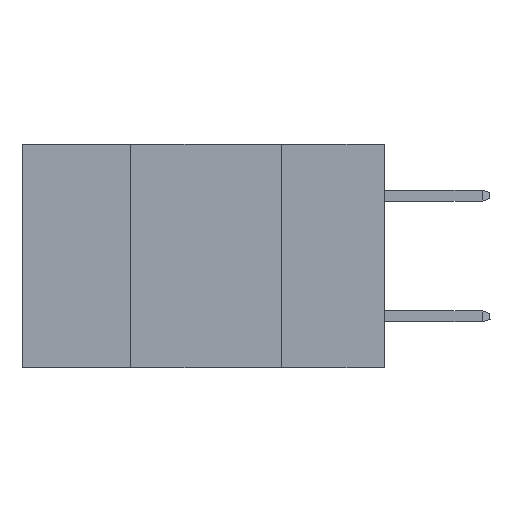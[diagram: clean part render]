
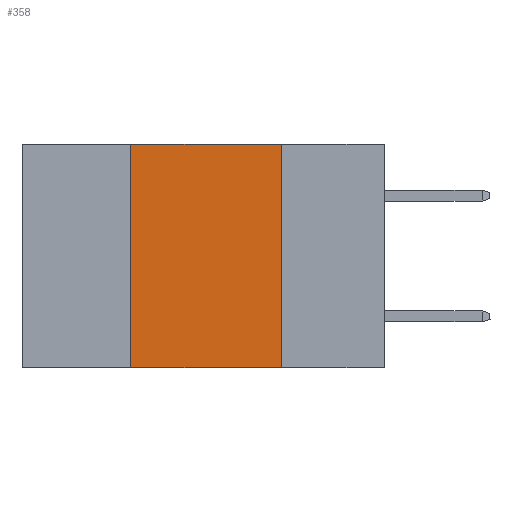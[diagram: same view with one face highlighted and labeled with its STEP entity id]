
A CAD part, left-side view. The second image highlights one B-rep face of the part: STEP entity #358.
In plain terms, the highlighted planar face has unit normal (-1, 0, 0).
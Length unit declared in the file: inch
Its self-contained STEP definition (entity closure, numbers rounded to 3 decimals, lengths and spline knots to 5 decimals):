
#71 = DIRECTION ( 'NONE',  ( 0., 0., -1. ) ) ;
#165 = CARTESIAN_POINT ( 'NONE',  ( 0., 0.42, -0.37 ) ) ;
#358 = ADVANCED_FACE ( 'NONE', ( #16092 ), #9782, .F. ) ;
#879 = VERTEX_POINT ( 'NONE', #4631 ) ;
#892 = DIRECTION ( 'NONE',  ( 0., -1., 0. ) ) ;
#1487 = CARTESIAN_POINT ( 'NONE',  ( 0., 0.17, -0.37 ) ) ;
#1535 = EDGE_CURVE ( 'NONE', #8017, #879, #15517, .T. ) ;
#1613 = DIRECTION ( 'NONE',  ( 0., 0., -1. ) ) ;
#1694 = AXIS2_PLACEMENT_3D ( 'NONE', #3619, #3434, #1613 ) ;
#3205 = EDGE_LOOP ( 'NONE', ( #7419, #20778, #12257, #13271 ) ) ;
#3256 = CARTESIAN_POINT ( 'NONE',  ( 0., 0.6, 0. ) ) ;
#3434 = DIRECTION ( 'NONE',  ( 1., 0., 0. ) ) ;
#3619 = CARTESIAN_POINT ( 'NONE',  ( 0., 0.6, 0. ) ) ;
#3693 = LINE ( 'NONE', #9057, #10819 ) ;
#4631 = CARTESIAN_POINT ( 'NONE',  ( 0., 0.42, 0. ) ) ;
#4871 = EDGE_CURVE ( 'NONE', #8017, #16399, #3693, .T. ) ;
#4913 = DIRECTION ( 'NONE',  ( 0., -1., 0. ) ) ;
#5069 = CARTESIAN_POINT ( 'NONE',  ( 0., 0.17, 0. ) ) ;
#6663 = CARTESIAN_POINT ( 'NONE',  ( 0., 0.17, -0.37 ) ) ;
#7247 = LINE ( 'NONE', #3256, #15378 ) ;
#7419 = ORIENTED_EDGE ( 'NONE', *, *, #15073, .F. ) ;
#8017 = VERTEX_POINT ( 'NONE', #20681 ) ;
#9057 = CARTESIAN_POINT ( 'NONE',  ( 0., 0.6, -0.37 ) ) ;
#9782 = PLANE ( 'NONE',  #1694 ) ;
#10819 = VECTOR ( 'NONE', #892, 39.37008 ) ;
#11705 = VECTOR ( 'NONE', #71, 39.37008 ) ;
#11714 = VECTOR ( 'NONE', #20709, 39.37008 ) ;
#12257 = ORIENTED_EDGE ( 'NONE', *, *, #1535, .F. ) ;
#13271 = ORIENTED_EDGE ( 'NONE', *, *, #4871, .T. ) ;
#15073 = EDGE_CURVE ( 'NONE', #15755, #16399, #16511, .T. ) ;
#15378 = VECTOR ( 'NONE', #4913, 39.37008 ) ;
#15517 = LINE ( 'NONE', #165, #11714 ) ;
#15755 = VERTEX_POINT ( 'NONE', #5069 ) ;
#16092 = FACE_OUTER_BOUND ( 'NONE', #3205, .T. ) ;
#16399 = VERTEX_POINT ( 'NONE', #1487 ) ;
#16511 = LINE ( 'NONE', #6663, #11705 ) ;
#18299 = EDGE_CURVE ( 'NONE', #879, #15755, #7247, .T. ) ;
#20681 = CARTESIAN_POINT ( 'NONE',  ( 0., 0.42, -0.37 ) ) ;
#20709 = DIRECTION ( 'NONE',  ( 0., 0., 1. ) ) ;
#20778 = ORIENTED_EDGE ( 'NONE', *, *, #18299, .F. ) ;
